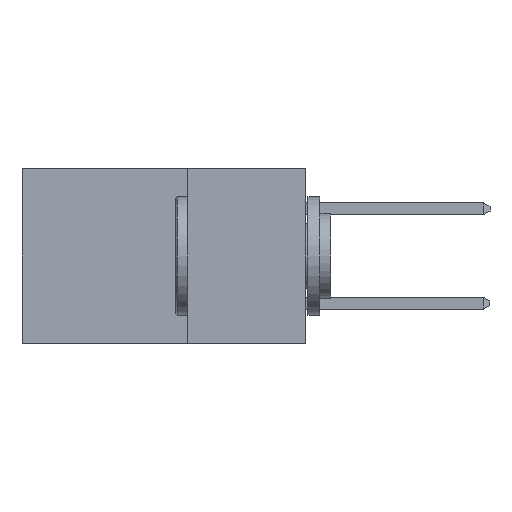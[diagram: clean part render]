
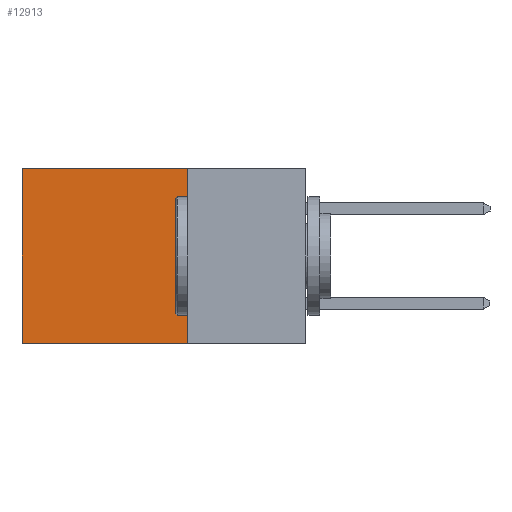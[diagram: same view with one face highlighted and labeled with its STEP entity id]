
A CAD part, left-side view. The second image highlights one B-rep face of the part: STEP entity #12913.
In plain terms, the highlighted planar face has unit normal (-1, 0, 0).
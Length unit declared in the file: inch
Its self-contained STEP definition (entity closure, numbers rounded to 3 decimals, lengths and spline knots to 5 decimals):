
#66 = CARTESIAN_POINT ( 'NONE',  ( 0.298, 0.6, 0. ) ) ;
#226 = DIRECTION ( 'NONE',  ( 0., 0., -1. ) ) ;
#1129 = DIRECTION ( 'NONE',  ( 1., 0., 0. ) ) ;
#1631 = CARTESIAN_POINT ( 'NONE',  ( 0.298, 0.25, 0. ) ) ;
#1853 = ORIENTED_EDGE ( 'NONE', *, *, #4529, .F. ) ;
#2498 = AXIS2_PLACEMENT_3D ( 'NONE', #21756, #1129, #13228 ) ;
#2740 = PLANE ( 'NONE',  #2498 ) ;
#3142 = VERTEX_POINT ( 'NONE', #16479 ) ;
#3866 = EDGE_CURVE ( 'NONE', #3142, #6504, #10033, .T. ) ;
#4309 = VECTOR ( 'NONE', #11373, 39.37008 ) ;
#4529 = EDGE_CURVE ( 'NONE', #9417, #20980, #10597, .T. ) ;
#6504 = VERTEX_POINT ( 'NONE', #11376 ) ;
#7857 = EDGE_CURVE ( 'NONE', #20980, #6504, #15985, .T. ) ;
#8479 = EDGE_CURVE ( 'NONE', #9417, #3142, #17596, .T. ) ;
#8814 = CARTESIAN_POINT ( 'NONE',  ( 0.298, 0.25, -0.37 ) ) ;
#9417 = VERTEX_POINT ( 'NONE', #1631 ) ;
#10033 = LINE ( 'NONE', #66, #14105 ) ;
#10547 = CARTESIAN_POINT ( 'NONE',  ( 0.298, 0.25, 0. ) ) ;
#10597 = LINE ( 'NONE', #10547, #19756 ) ;
#11373 = DIRECTION ( 'NONE',  ( 0., 1., 0. ) ) ;
#11376 = CARTESIAN_POINT ( 'NONE',  ( 0.298, 0.6, -0.37 ) ) ;
#11420 = VECTOR ( 'NONE', #18691, 39.37008 ) ;
#11458 = EDGE_LOOP ( 'NONE', ( #16685, #16515, #1853, #21577 ) ) ;
#12913 = ADVANCED_FACE ( 'NONE', ( #13425 ), #2740, .F. ) ;
#13228 = DIRECTION ( 'NONE',  ( 0., 0., -1. ) ) ;
#13271 = DIRECTION ( 'NONE',  ( 0., 0., -1. ) ) ;
#13425 = FACE_OUTER_BOUND ( 'NONE', #11458, .T. ) ;
#14105 = VECTOR ( 'NONE', #226, 39.37008 ) ;
#15985 = LINE ( 'NONE', #16207, #11420 ) ;
#16207 = CARTESIAN_POINT ( 'NONE',  ( 0.298, 0.25, -0.37 ) ) ;
#16479 = CARTESIAN_POINT ( 'NONE',  ( 0.298, 0.6, 0. ) ) ;
#16515 = ORIENTED_EDGE ( 'NONE', *, *, #7857, .F. ) ;
#16685 = ORIENTED_EDGE ( 'NONE', *, *, #3866, .T. ) ;
#17596 = LINE ( 'NONE', #21643, #4309 ) ;
#18691 = DIRECTION ( 'NONE',  ( 0., 1., 0. ) ) ;
#19756 = VECTOR ( 'NONE', #13271, 39.37008 ) ;
#20980 = VERTEX_POINT ( 'NONE', #8814 ) ;
#21577 = ORIENTED_EDGE ( 'NONE', *, *, #8479, .T. ) ;
#21643 = CARTESIAN_POINT ( 'NONE',  ( 0.298, 0.25, 0. ) ) ;
#21756 = CARTESIAN_POINT ( 'NONE',  ( 0.298, 0.25, 0. ) ) ;
